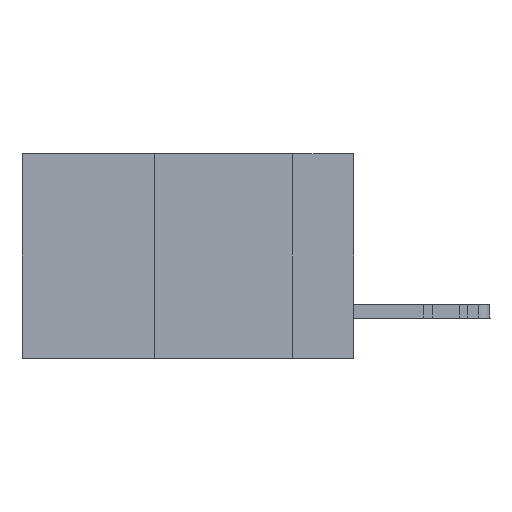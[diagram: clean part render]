
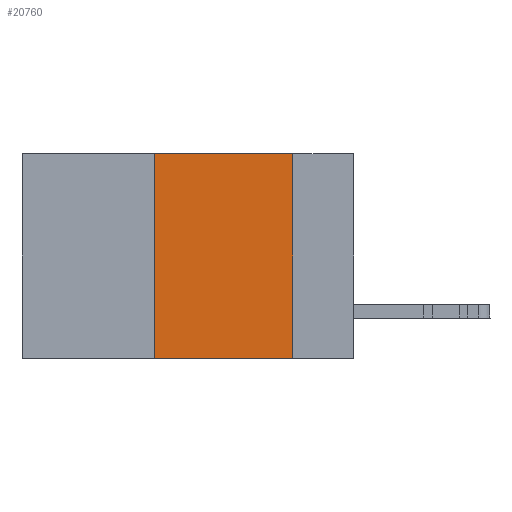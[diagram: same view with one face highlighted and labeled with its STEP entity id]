
A CAD part, left-side view. The second image highlights one B-rep face of the part: STEP entity #20760.
In plain terms, the highlighted planar face has unit normal (-1, 0, 0).
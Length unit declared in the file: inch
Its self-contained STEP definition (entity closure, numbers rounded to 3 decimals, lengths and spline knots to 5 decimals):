
#5456 = VERTEX_POINT ( 'NONE', #39997 ) ;
#5955 = ORIENTED_EDGE ( 'NONE', *, *, #16089, .T. ) ;
#6537 = LINE ( 'NONE', #10294, #39475 ) ;
#6797 = AXIS2_PLACEMENT_3D ( 'NONE', #7561, #30368, #10704 ) ;
#7360 = ORIENTED_EDGE ( 'NONE', *, *, #8245, .F. ) ;
#7538 = EDGE_LOOP ( 'NONE', ( #17042, #7360, #26997, #5955 ) ) ;
#7561 = CARTESIAN_POINT ( 'NONE',  ( 0., 0.6, 0. ) ) ;
#7575 = DIRECTION ( 'NONE',  ( 0., 0., 1. ) ) ;
#8245 = EDGE_CURVE ( 'NONE', #10707, #38648, #27779, .T. ) ;
#10294 = CARTESIAN_POINT ( 'NONE',  ( 0., 0.11, 0. ) ) ;
#10519 = CARTESIAN_POINT ( 'NONE',  ( 0., 0.36, 0. ) ) ;
#10704 = DIRECTION ( 'NONE',  ( 0., 0., -1. ) ) ;
#10707 = VERTEX_POINT ( 'NONE', #34291 ) ;
#10802 = VECTOR ( 'NONE', #21466, 39.37008 ) ;
#13414 = VECTOR ( 'NONE', #7575, 39.37008 ) ;
#13449 = LINE ( 'NONE', #10519, #13414 ) ;
#15636 = DIRECTION ( 'NONE',  ( 0., -1., 0. ) ) ;
#16089 = EDGE_CURVE ( 'NONE', #5456, #17446, #37377, .T. ) ;
#16809 = CARTESIAN_POINT ( 'NONE',  ( 0., 0.11, 0. ) ) ;
#17042 = ORIENTED_EDGE ( 'NONE', *, *, #19550, .F. ) ;
#17209 = PLANE ( 'NONE',  #6797 ) ;
#17446 = VERTEX_POINT ( 'NONE', #24824 ) ;
#19550 = EDGE_CURVE ( 'NONE', #38648, #17446, #6537, .T. ) ;
#20760 = ADVANCED_FACE ( 'NONE', ( #24086 ), #17209, .F. ) ;
#21118 = VECTOR ( 'NONE', #15636, 39.37008 ) ;
#21290 = CARTESIAN_POINT ( 'NONE',  ( 0., 0.6, 0. ) ) ;
#21466 = DIRECTION ( 'NONE',  ( 0., -1., 0. ) ) ;
#24086 = FACE_OUTER_BOUND ( 'NONE', #7538, .T. ) ;
#24824 = CARTESIAN_POINT ( 'NONE',  ( 0., 0.11, -0.37 ) ) ;
#26401 = DIRECTION ( 'NONE',  ( 0., 0., -1. ) ) ;
#26997 = ORIENTED_EDGE ( 'NONE', *, *, #36046, .F. ) ;
#27779 = LINE ( 'NONE', #21290, #21118 ) ;
#30368 = DIRECTION ( 'NONE',  ( 1., 0., 0. ) ) ;
#34291 = CARTESIAN_POINT ( 'NONE',  ( 0., 0.36, 0. ) ) ;
#36046 = EDGE_CURVE ( 'NONE', #5456, #10707, #13449, .T. ) ;
#36766 = CARTESIAN_POINT ( 'NONE',  ( 0., 0.6, -0.37 ) ) ;
#37377 = LINE ( 'NONE', #36766, #10802 ) ;
#38648 = VERTEX_POINT ( 'NONE', #16809 ) ;
#39475 = VECTOR ( 'NONE', #26401, 39.37008 ) ;
#39997 = CARTESIAN_POINT ( 'NONE',  ( 0., 0.36, -0.37 ) ) ;
